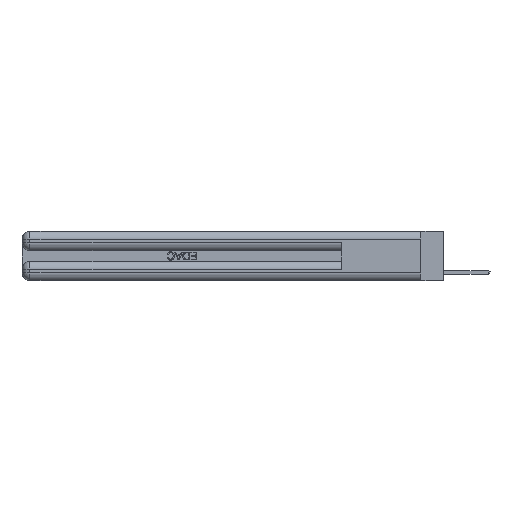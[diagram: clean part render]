
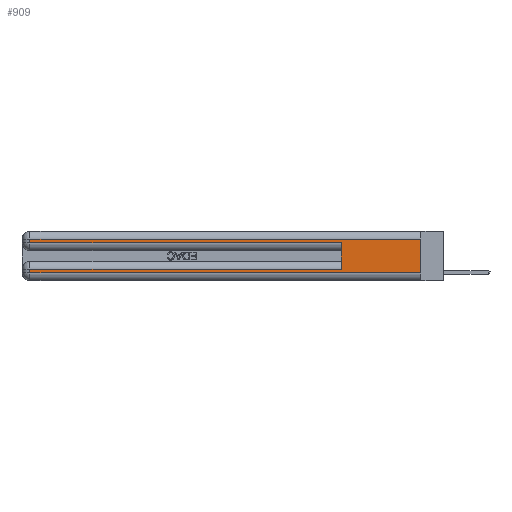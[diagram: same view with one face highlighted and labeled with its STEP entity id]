
A CAD part, left-side view. The second image highlights one B-rep face of the part: STEP entity #909.
In plain terms, the highlighted planar face has unit normal (-1, 0, 0).
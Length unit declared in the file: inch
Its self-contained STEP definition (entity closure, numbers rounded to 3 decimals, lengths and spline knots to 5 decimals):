
#433 = VERTEX_POINT ( 'NONE', #15070 ) ;
#909 = ADVANCED_FACE ( 'NONE', ( #8583 ), #19227, .F. ) ;
#1165 = CARTESIAN_POINT ( 'NONE',  ( 0., 0., 0.285 ) ) ;
#2185 = CARTESIAN_POINT ( 'NONE',  ( 0., 0., 0.06 ) ) ;
#3045 = ORIENTED_EDGE ( 'NONE', *, *, #28286, .T. ) ;
#3194 = CARTESIAN_POINT ( 'NONE',  ( 0., 2.94, 0.37 ) ) ;
#3288 = ORIENTED_EDGE ( 'NONE', *, *, #15681, .F. ) ;
#3591 = DIRECTION ( 'NONE',  ( 1., 0., 0. ) ) ;
#3605 = ORIENTED_EDGE ( 'NONE', *, *, #10600, .T. ) ;
#3801 = DIRECTION ( 'NONE',  ( 0., 0., -1. ) ) ;
#5136 = CARTESIAN_POINT ( 'NONE',  ( 0., 0., 0.31 ) ) ;
#5270 = ORIENTED_EDGE ( 'NONE', *, *, #7493, .T. ) ;
#5785 = CARTESIAN_POINT ( 'NONE',  ( 0., 0.6, 0.145 ) ) ;
#6583 = CARTESIAN_POINT ( 'NONE',  ( 0., 0., 0.37 ) ) ;
#6778 = CARTESIAN_POINT ( 'NONE',  ( 0., 0.6, 0.285 ) ) ;
#7287 = VECTOR ( 'NONE', #21883, 39.37008 ) ;
#7493 = EDGE_CURVE ( 'NONE', #23339, #17025, #10676, .T. ) ;
#8192 = DIRECTION ( 'NONE',  ( 0., 0., -1. ) ) ;
#8303 = VECTOR ( 'NONE', #8192, 39.37008 ) ;
#8383 = EDGE_CURVE ( 'NONE', #17025, #25237, #25379, .T. ) ;
#8583 = FACE_OUTER_BOUND ( 'NONE', #29899, .T. ) ;
#8903 = VERTEX_POINT ( 'NONE', #16207 ) ;
#10063 = CARTESIAN_POINT ( 'NONE',  ( 0., 0., 0.06 ) ) ;
#10244 = ORIENTED_EDGE ( 'NONE', *, *, #31562, .F. ) ;
#10600 = EDGE_CURVE ( 'NONE', #8903, #23431, #29414, .T. ) ;
#10653 = VECTOR ( 'NONE', #26653, 39.37008 ) ;
#10676 = LINE ( 'NONE', #3194, #8303 ) ;
#13441 = VECTOR ( 'NONE', #26813, 39.37008 ) ;
#14918 = VERTEX_POINT ( 'NONE', #10063 ) ;
#15067 = CARTESIAN_POINT ( 'NONE',  ( 0., 0., 0.31 ) ) ;
#15070 = CARTESIAN_POINT ( 'NONE',  ( 0., 0.6, 0.085 ) ) ;
#15269 = AXIS2_PLACEMENT_3D ( 'NONE', #26655, #3591, #3801 ) ;
#15681 = EDGE_CURVE ( 'NONE', #18849, #14918, #25155, .T. ) ;
#15844 = VECTOR ( 'NONE', #31184, 39.37008 ) ;
#15883 = ORIENTED_EDGE ( 'NONE', *, *, #17919, .T. ) ;
#16207 = CARTESIAN_POINT ( 'NONE',  ( 0., 2.94, 0.085 ) ) ;
#17025 = VERTEX_POINT ( 'NONE', #27795 ) ;
#17439 = DIRECTION ( 'NONE',  ( 0., 0., -1. ) ) ;
#17519 = LINE ( 'NONE', #15067, #20673 ) ;
#17919 = EDGE_CURVE ( 'NONE', #433, #8903, #21326, .T. ) ;
#17937 = DIRECTION ( 'NONE',  ( 0., 1., 0. ) ) ;
#18516 = ORIENTED_EDGE ( 'NONE', *, *, #26954, .T. ) ;
#18849 = VERTEX_POINT ( 'NONE', #5136 ) ;
#19227 = PLANE ( 'NONE',  #15269 ) ;
#20673 = VECTOR ( 'NONE', #17937, 39.37008 ) ;
#21326 = LINE ( 'NONE', #24384, #13441 ) ;
#21883 = DIRECTION ( 'NONE',  ( 0., 0., -1. ) ) ;
#23084 = VECTOR ( 'NONE', #17439, 39.37008 ) ;
#23339 = VERTEX_POINT ( 'NONE', #32550 ) ;
#23431 = VERTEX_POINT ( 'NONE', #25567 ) ;
#23777 = LINE ( 'NONE', #5785, #15844 ) ;
#24089 = ORIENTED_EDGE ( 'NONE', *, *, #8383, .T. ) ;
#24234 = VECTOR ( 'NONE', #25139, 39.37008 ) ;
#24384 = CARTESIAN_POINT ( 'NONE',  ( 0., 0., 0.085 ) ) ;
#25139 = DIRECTION ( 'NONE',  ( 0., -1., 0. ) ) ;
#25155 = LINE ( 'NONE', #6583, #7287 ) ;
#25237 = VERTEX_POINT ( 'NONE', #6778 ) ;
#25379 = LINE ( 'NONE', #1165, #10653 ) ;
#25567 = CARTESIAN_POINT ( 'NONE',  ( 0., 2.94, 0.06 ) ) ;
#26653 = DIRECTION ( 'NONE',  ( 0., -1., 0. ) ) ;
#26655 = CARTESIAN_POINT ( 'NONE',  ( 0., 0., 0.37 ) ) ;
#26813 = DIRECTION ( 'NONE',  ( 0., 1., 0. ) ) ;
#26954 = EDGE_CURVE ( 'NONE', #18849, #23339, #17519, .T. ) ;
#27795 = CARTESIAN_POINT ( 'NONE',  ( 0., 2.94, 0.285 ) ) ;
#28286 = EDGE_CURVE ( 'NONE', #23431, #14918, #32135, .T. ) ;
#29414 = LINE ( 'NONE', #32705, #23084 ) ;
#29899 = EDGE_LOOP ( 'NONE', ( #3288, #18516, #5270, #24089, #10244, #15883, #3605, #3045 ) ) ;
#31184 = DIRECTION ( 'NONE',  ( 0., 0., 1. ) ) ;
#31562 = EDGE_CURVE ( 'NONE', #433, #25237, #23777, .T. ) ;
#32135 = LINE ( 'NONE', #2185, #24234 ) ;
#32550 = CARTESIAN_POINT ( 'NONE',  ( 0., 2.94, 0.31 ) ) ;
#32705 = CARTESIAN_POINT ( 'NONE',  ( 0., 2.94, 0.37 ) ) ;
